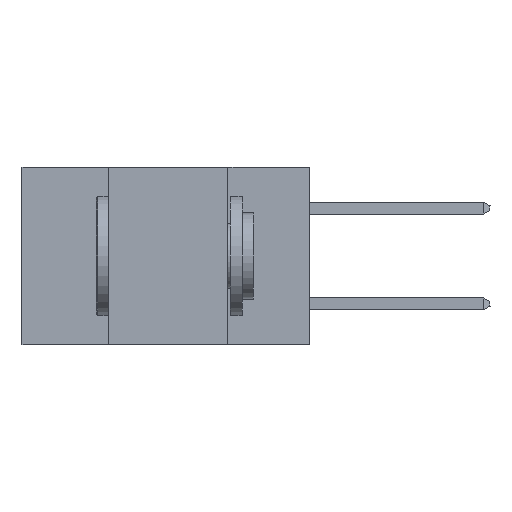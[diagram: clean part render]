
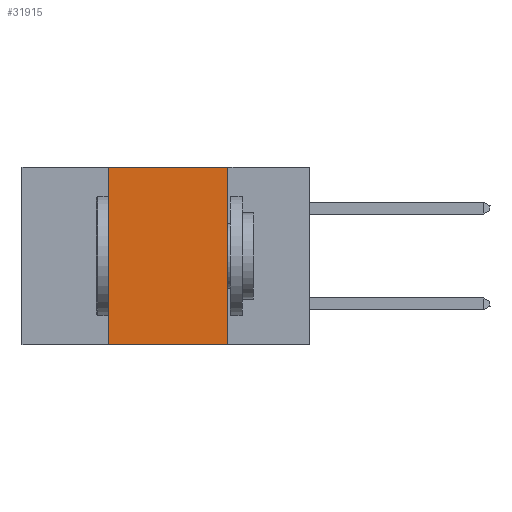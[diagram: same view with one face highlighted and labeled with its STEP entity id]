
A CAD part, left-side view. The second image highlights one B-rep face of the part: STEP entity #31915.
In plain terms, the highlighted planar face has unit normal (-1, 0, 0).
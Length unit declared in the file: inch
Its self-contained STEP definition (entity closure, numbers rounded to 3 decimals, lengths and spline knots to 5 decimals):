
#870 = VERTEX_POINT ( 'NONE', #25722 ) ;
#919 = ORIENTED_EDGE ( 'NONE', *, *, #964, .F. ) ;
#964 = EDGE_CURVE ( 'NONE', #29296, #870, #11959, .T. ) ;
#1186 = CARTESIAN_POINT ( 'NONE',  ( 0., 0.6, 0. ) ) ;
#3502 = DIRECTION ( 'NONE',  ( 1., 0., 0. ) ) ;
#3997 = VERTEX_POINT ( 'NONE', #26719 ) ;
#4161 = ORIENTED_EDGE ( 'NONE', *, *, #17260, .T. ) ;
#4655 = CARTESIAN_POINT ( 'NONE',  ( 0., 0.17, 0. ) ) ;
#5385 = DIRECTION ( 'NONE',  ( 0., -1., 0. ) ) ;
#5495 = CARTESIAN_POINT ( 'NONE',  ( 0., 0.6, -0.37 ) ) ;
#5660 = CARTESIAN_POINT ( 'NONE',  ( 0., 0.17, 0. ) ) ;
#7173 = DIRECTION ( 'NONE',  ( 0., 0., -1. ) ) ;
#9461 = EDGE_CURVE ( 'NONE', #3997, #29296, #26585, .T. ) ;
#11536 = VECTOR ( 'NONE', #31358, 39.37008 ) ;
#11959 = LINE ( 'NONE', #4655, #18264 ) ;
#12092 = EDGE_LOOP ( 'NONE', ( #919, #14569, #23306, #4161 ) ) ;
#14569 = ORIENTED_EDGE ( 'NONE', *, *, #9461, .F. ) ;
#14700 = FACE_OUTER_BOUND ( 'NONE', #12092, .T. ) ;
#15868 = LINE ( 'NONE', #25893, #11536 ) ;
#16125 = DIRECTION ( 'NONE',  ( 0., 0., -1. ) ) ;
#17260 = EDGE_CURVE ( 'NONE', #27636, #870, #23795, .T. ) ;
#18264 = VECTOR ( 'NONE', #7173, 39.37008 ) ;
#18454 = CARTESIAN_POINT ( 'NONE',  ( 0., 0.42, -0.37 ) ) ;
#19606 = VECTOR ( 'NONE', #25813, 39.37008 ) ;
#20813 = CARTESIAN_POINT ( 'NONE',  ( 0., 0.6, 0. ) ) ;
#22851 = AXIS2_PLACEMENT_3D ( 'NONE', #1186, #3502, #16125 ) ;
#23306 = ORIENTED_EDGE ( 'NONE', *, *, #27044, .F. ) ;
#23387 = VECTOR ( 'NONE', #5385, 39.37008 ) ;
#23795 = LINE ( 'NONE', #5495, #23387 ) ;
#25722 = CARTESIAN_POINT ( 'NONE',  ( 0., 0.17, -0.37 ) ) ;
#25813 = DIRECTION ( 'NONE',  ( 0., -1., 0. ) ) ;
#25893 = CARTESIAN_POINT ( 'NONE',  ( 0., 0.42, 0. ) ) ;
#26585 = LINE ( 'NONE', #20813, #19606 ) ;
#26719 = CARTESIAN_POINT ( 'NONE',  ( 0., 0.42, 0. ) ) ;
#27044 = EDGE_CURVE ( 'NONE', #27636, #3997, #15868, .T. ) ;
#27636 = VERTEX_POINT ( 'NONE', #18454 ) ;
#28582 = PLANE ( 'NONE',  #22851 ) ;
#29296 = VERTEX_POINT ( 'NONE', #5660 ) ;
#31358 = DIRECTION ( 'NONE',  ( 0., 0., 1. ) ) ;
#31915 = ADVANCED_FACE ( 'NONE', ( #14700 ), #28582, .F. ) ;
